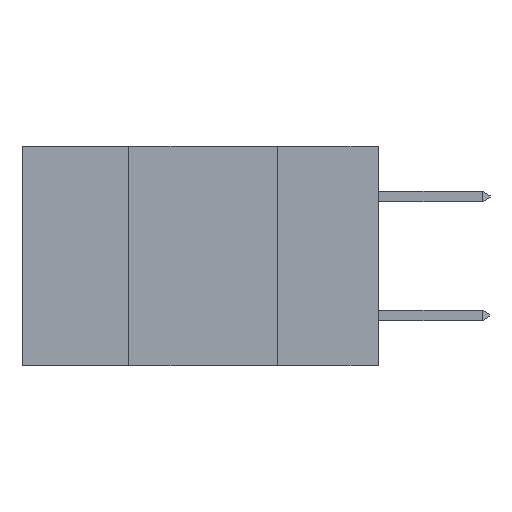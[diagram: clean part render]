
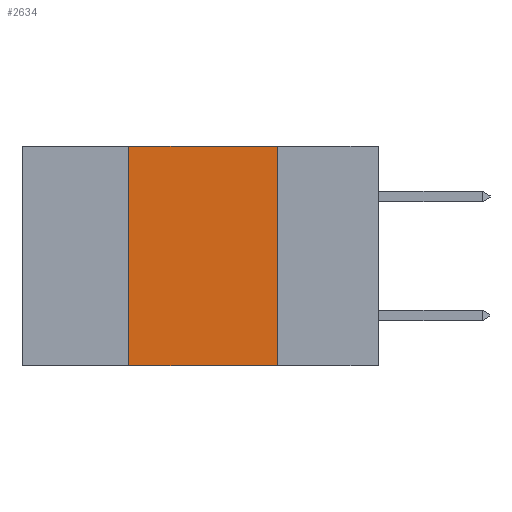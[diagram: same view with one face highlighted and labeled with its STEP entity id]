
A CAD part, left-side view. The second image highlights one B-rep face of the part: STEP entity #2634.
In plain terms, the highlighted planar face has unit normal (-1, 0, 0).
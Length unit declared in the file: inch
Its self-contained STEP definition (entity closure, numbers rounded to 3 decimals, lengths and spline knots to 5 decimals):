
#521 = LINE ( 'NONE', #4254, #11886 ) ;
#726 = DIRECTION ( 'NONE',  ( 0., -1., 0. ) ) ;
#918 = VECTOR ( 'NONE', #5779, 39.37008 ) ;
#922 = LINE ( 'NONE', #10521, #12263 ) ;
#1081 = PLANE ( 'NONE',  #8960 ) ;
#2634 = ADVANCED_FACE ( 'NONE', ( #12886 ), #1081, .F. ) ;
#2723 = ORIENTED_EDGE ( 'NONE', *, *, #10391, .F. ) ;
#2785 = VERTEX_POINT ( 'NONE', #12033 ) ;
#2997 = CARTESIAN_POINT ( 'NONE',  ( 0., 0.42, -0.37 ) ) ;
#3258 = VERTEX_POINT ( 'NONE', #13964 ) ;
#3367 = CARTESIAN_POINT ( 'NONE',  ( 0., 0.6, 0. ) ) ;
#4254 = CARTESIAN_POINT ( 'NONE',  ( 0., 0.6, -0.37 ) ) ;
#5369 = VERTEX_POINT ( 'NONE', #6544 ) ;
#5779 = DIRECTION ( 'NONE',  ( 0., 0., 1. ) ) ;
#5877 = CARTESIAN_POINT ( 'NONE',  ( 0., 0.42, 0. ) ) ;
#5982 = EDGE_CURVE ( 'NONE', #5369, #3258, #11378, .T. ) ;
#6082 = DIRECTION ( 'NONE',  ( 0., 0., -1. ) ) ;
#6544 = CARTESIAN_POINT ( 'NONE',  ( 0., 0.17, 0. ) ) ;
#8444 = ORIENTED_EDGE ( 'NONE', *, *, #5982, .F. ) ;
#8789 = ORIENTED_EDGE ( 'NONE', *, *, #13282, .T. ) ;
#8960 = AXIS2_PLACEMENT_3D ( 'NONE', #3367, #12300, #6082 ) ;
#9369 = ORIENTED_EDGE ( 'NONE', *, *, #12039, .F. ) ;
#9839 = LINE ( 'NONE', #5877, #918 ) ;
#10391 = EDGE_CURVE ( 'NONE', #12129, #2785, #9839, .T. ) ;
#10521 = CARTESIAN_POINT ( 'NONE',  ( 0., 0.6, 0. ) ) ;
#11378 = LINE ( 'NONE', #14017, #13750 ) ;
#11748 = EDGE_LOOP ( 'NONE', ( #8444, #9369, #2723, #8789 ) ) ;
#11886 = VECTOR ( 'NONE', #726, 39.37008 ) ;
#12033 = CARTESIAN_POINT ( 'NONE',  ( 0., 0.42, 0. ) ) ;
#12039 = EDGE_CURVE ( 'NONE', #2785, #5369, #922, .T. ) ;
#12129 = VERTEX_POINT ( 'NONE', #2997 ) ;
#12263 = VECTOR ( 'NONE', #12582, 39.37008 ) ;
#12300 = DIRECTION ( 'NONE',  ( 1., 0., 0. ) ) ;
#12305 = DIRECTION ( 'NONE',  ( 0., 0., -1. ) ) ;
#12582 = DIRECTION ( 'NONE',  ( 0., -1., 0. ) ) ;
#12886 = FACE_OUTER_BOUND ( 'NONE', #11748, .T. ) ;
#13282 = EDGE_CURVE ( 'NONE', #12129, #3258, #521, .T. ) ;
#13750 = VECTOR ( 'NONE', #12305, 39.37008 ) ;
#13964 = CARTESIAN_POINT ( 'NONE',  ( 0., 0.17, -0.37 ) ) ;
#14017 = CARTESIAN_POINT ( 'NONE',  ( 0., 0.17, 0. ) ) ;
